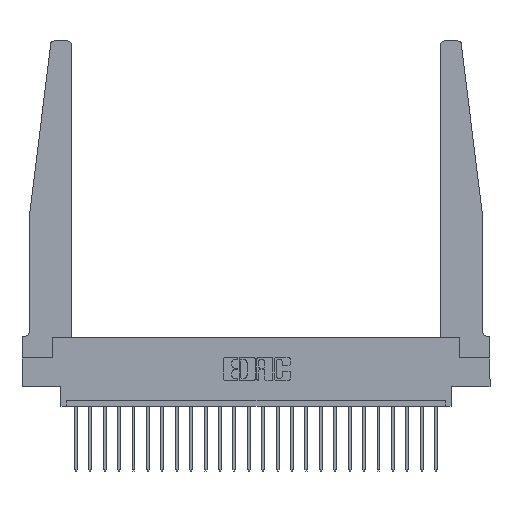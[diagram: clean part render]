
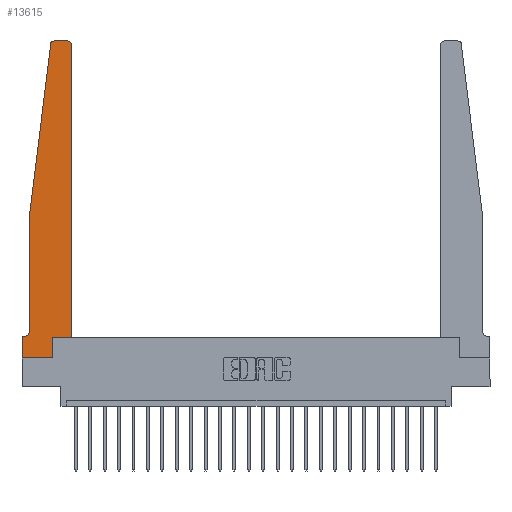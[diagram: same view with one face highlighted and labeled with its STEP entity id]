
A CAD part, top view. The second image highlights one B-rep face of the part: STEP entity #13615.
In plain terms, the highlighted planar face has unit normal (0, 0, 1).
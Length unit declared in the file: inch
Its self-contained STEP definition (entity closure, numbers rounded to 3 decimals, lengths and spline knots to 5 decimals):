
#183 = DIRECTION ( 'NONE',  ( 0., -1., 0. ) ) ;
#192 = DIRECTION ( 'NONE',  ( -1., 0., 0. ) ) ;
#229 = ORIENTED_EDGE ( 'NONE', *, *, #11737, .T. ) ;
#679 = CARTESIAN_POINT ( 'NONE',  ( 0.065, 0.2375, 0.37 ) ) ;
#807 = CARTESIAN_POINT ( 'NONE',  ( 0.395, 2.72, 0.37 ) ) ;
#1219 = ORIENTED_EDGE ( 'NONE', *, *, #2650, .T. ) ;
#1365 = FACE_OUTER_BOUND ( 'NONE', #7556, .T. ) ;
#1380 = LINE ( 'NONE', #15550, #5618 ) ;
#1490 = VECTOR ( 'NONE', #192, 39.37008 ) ;
#1957 = DIRECTION ( 'NONE',  ( 1., 0., 0. ) ) ;
#1988 = DIRECTION ( 'NONE',  ( -1., 0., 0. ) ) ;
#2604 = DIRECTION ( 'NONE',  ( 0., 0., 1. ) ) ;
#2650 = EDGE_CURVE ( 'NONE', #20532, #17191, #20445, .T. ) ;
#2909 = CARTESIAN_POINT ( 'NONE',  ( 0.425, 0.18, 0.37 ) ) ;
#3036 = VECTOR ( 'NONE', #1957, 39.37008 ) ;
#3327 = CARTESIAN_POINT ( 'NONE',  ( 0.395, 2.75, 0.37 ) ) ;
#3951 = EDGE_CURVE ( 'NONE', #9373, #13495, #19541, .T. ) ;
#4016 = EDGE_CURVE ( 'NONE', #18828, #20532, #17010, .T. ) ;
#4024 = EDGE_CURVE ( 'NONE', #17282, #6730, #17296, .T. ) ;
#4542 = VECTOR ( 'NONE', #11615, 39.37008 ) ;
#4964 = LINE ( 'NONE', #19486, #16675 ) ;
#4972 = CARTESIAN_POINT ( 'NONE',  ( 0., 0.1875, 0.37 ) ) ;
#5430 = EDGE_CURVE ( 'NONE', #13495, #12772, #1380, .T. ) ;
#5485 = VERTEX_POINT ( 'NONE', #3327 ) ;
#5618 = VECTOR ( 'NONE', #6689, 39.37008 ) ;
#5638 = ORIENTED_EDGE ( 'NONE', *, *, #21449, .T. ) ;
#5728 = CARTESIAN_POINT ( 'NONE',  ( 0.065, 1.25, 0.37 ) ) ;
#5883 = DIRECTION ( 'NONE',  ( 1., 0., 0. ) ) ;
#6174 = ORIENTED_EDGE ( 'NONE', *, *, #4024, .T. ) ;
#6452 = CARTESIAN_POINT ( 'NONE',  ( 0.2605, 0., 0.37 ) ) ;
#6489 = CARTESIAN_POINT ( 'NONE',  ( 0., 0., 0.37 ) ) ;
#6689 = DIRECTION ( 'NONE',  ( 0., 1., 0. ) ) ;
#6730 = VERTEX_POINT ( 'NONE', #6452 ) ;
#7048 = DIRECTION ( 'NONE',  ( 1., 0., 0. ) ) ;
#7556 = EDGE_LOOP ( 'NONE', ( #8308, #16500, #20259, #1219, #13844, #9908, #5638, #6174, #16773, #13637, #19755, #229 ) ) ;
#7614 = LINE ( 'NONE', #11450, #4542 ) ;
#7923 = CIRCLE ( 'NONE', #18237, 0.05 ) ;
#8308 = ORIENTED_EDGE ( 'NONE', *, *, #10867, .T. ) ;
#8776 = DIRECTION ( 'NONE',  ( 0., 1., 0. ) ) ;
#9373 = VERTEX_POINT ( 'NONE', #22354 ) ;
#9444 = DIRECTION ( 'NONE',  ( 0., 0., 1. ) ) ;
#9621 = CARTESIAN_POINT ( 'NONE',  ( 0., 0., 0.37 ) ) ;
#9778 = DIRECTION ( 'NONE',  ( 1., 0., 0. ) ) ;
#9908 = ORIENTED_EDGE ( 'NONE', *, *, #21655, .T. ) ;
#10127 = CIRCLE ( 'NONE', #10985, 0.03 ) ;
#10674 = AXIS2_PLACEMENT_3D ( 'NONE', #22659, #18977, #7048 ) ;
#10824 = CARTESIAN_POINT ( 'NONE',  ( 0.015, 0.2375, 0.37 ) ) ;
#10867 = EDGE_CURVE ( 'NONE', #5485, #18682, #7614, .T. ) ;
#10943 = CARTESIAN_POINT ( 'NONE',  ( 0.065, 0.1875, 0.37 ) ) ;
#10957 = CIRCLE ( 'NONE', #10674, 0.03 ) ;
#10959 = CARTESIAN_POINT ( 'NONE',  ( 0.425, 2.72, 0.37 ) ) ;
#10985 = AXIS2_PLACEMENT_3D ( 'NONE', #807, #2604, #22551 ) ;
#11020 = AXIS2_PLACEMENT_3D ( 'NONE', #12971, #9444, #5883 ) ;
#11053 = EDGE_CURVE ( 'NONE', #18682, #18828, #10957, .T. ) ;
#11253 = CARTESIAN_POINT ( 'NONE',  ( 0.27653, 2.75, 0.37 ) ) ;
#11450 = CARTESIAN_POINT ( 'NONE',  ( 0.25, 2.75, 0.37 ) ) ;
#11608 = VECTOR ( 'NONE', #17668, 39.37008 ) ;
#11615 = DIRECTION ( 'NONE',  ( -1., 0., 0. ) ) ;
#11737 = EDGE_CURVE ( 'NONE', #12772, #5485, #10127, .T. ) ;
#12772 = VERTEX_POINT ( 'NONE', #10959 ) ;
#12971 = CARTESIAN_POINT ( 'NONE',  ( 0., 0.1875, 0.37 ) ) ;
#13104 = VERTEX_POINT ( 'NONE', #4972 ) ;
#13495 = VERTEX_POINT ( 'NONE', #2909 ) ;
#13615 = ADVANCED_FACE ( 'NONE', ( #1365 ), #16470, .T. ) ;
#13637 = ORIENTED_EDGE ( 'NONE', *, *, #3951, .T. ) ;
#13826 = CARTESIAN_POINT ( 'NONE',  ( 0.015, 0.1875, 0.37 ) ) ;
#13844 = ORIENTED_EDGE ( 'NONE', *, *, #17624, .T. ) ;
#14306 = CARTESIAN_POINT ( 'NONE',  ( 0., 0., 0.37 ) ) ;
#14347 = DIRECTION ( 'NONE',  ( 0., 0., -1. ) ) ;
#14798 = VECTOR ( 'NONE', #183, 39.37008 ) ;
#15215 = EDGE_CURVE ( 'NONE', #6730, #9373, #4964, .T. ) ;
#15324 = VECTOR ( 'NONE', #9778, 39.37008 ) ;
#15347 = VERTEX_POINT ( 'NONE', #13826 ) ;
#15451 = CARTESIAN_POINT ( 'NONE',  ( 0.24675, 2.72367, 0.37 ) ) ;
#15550 = CARTESIAN_POINT ( 'NONE',  ( 0.425, 0.18, 0.37 ) ) ;
#16352 = LINE ( 'NONE', #14306, #11608 ) ;
#16470 = PLANE ( 'NONE',  #11020 ) ;
#16500 = ORIENTED_EDGE ( 'NONE', *, *, #11053, .T. ) ;
#16675 = VECTOR ( 'NONE', #8776, 39.37008 ) ;
#16773 = ORIENTED_EDGE ( 'NONE', *, *, #15215, .T. ) ;
#17010 = LINE ( 'NONE', #18674, #20674 ) ;
#17191 = VERTEX_POINT ( 'NONE', #679 ) ;
#17282 = VERTEX_POINT ( 'NONE', #6489 ) ;
#17296 = LINE ( 'NONE', #9621, #15324 ) ;
#17624 = EDGE_CURVE ( 'NONE', #17191, #15347, #7923, .T. ) ;
#17668 = DIRECTION ( 'NONE',  ( 0., -1., 0. ) ) ;
#18011 = LINE ( 'NONE', #10943, #1490 ) ;
#18237 = AXIS2_PLACEMENT_3D ( 'NONE', #10824, #14347, #1988 ) ;
#18674 = CARTESIAN_POINT ( 'NONE',  ( 0.065, 1.25, 0.37 ) ) ;
#18682 = VERTEX_POINT ( 'NONE', #11253 ) ;
#18828 = VERTEX_POINT ( 'NONE', #15451 ) ;
#18977 = DIRECTION ( 'NONE',  ( 0., 0., 1. ) ) ;
#19486 = CARTESIAN_POINT ( 'NONE',  ( 0.2605, 0.18, 0.37 ) ) ;
#19541 = LINE ( 'NONE', #19802, #3036 ) ;
#19755 = ORIENTED_EDGE ( 'NONE', *, *, #5430, .T. ) ;
#19802 = CARTESIAN_POINT ( 'NONE',  ( 0.425, 0.18, 0.37 ) ) ;
#20259 = ORIENTED_EDGE ( 'NONE', *, *, #4016, .T. ) ;
#20306 = CARTESIAN_POINT ( 'NONE',  ( 0.065, 1.25, 0.37 ) ) ;
#20445 = LINE ( 'NONE', #5728, #14798 ) ;
#20532 = VERTEX_POINT ( 'NONE', #20306 ) ;
#20674 = VECTOR ( 'NONE', #22065, 39.37008 ) ;
#21449 = EDGE_CURVE ( 'NONE', #13104, #17282, #16352, .T. ) ;
#21655 = EDGE_CURVE ( 'NONE', #15347, #13104, #18011, .T. ) ;
#22065 = DIRECTION ( 'NONE',  ( -0.122, -0.992, 0. ) ) ;
#22354 = CARTESIAN_POINT ( 'NONE',  ( 0.2605, 0.18, 0.37 ) ) ;
#22551 = DIRECTION ( 'NONE',  ( 1., 0., 0. ) ) ;
#22659 = CARTESIAN_POINT ( 'NONE',  ( 0.27653, 2.72, 0.37 ) ) ;
